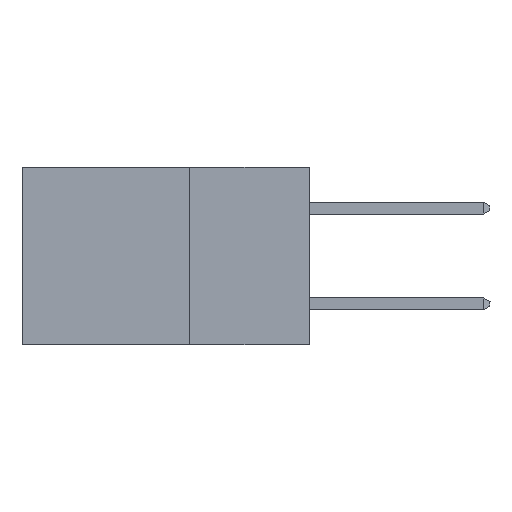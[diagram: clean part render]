
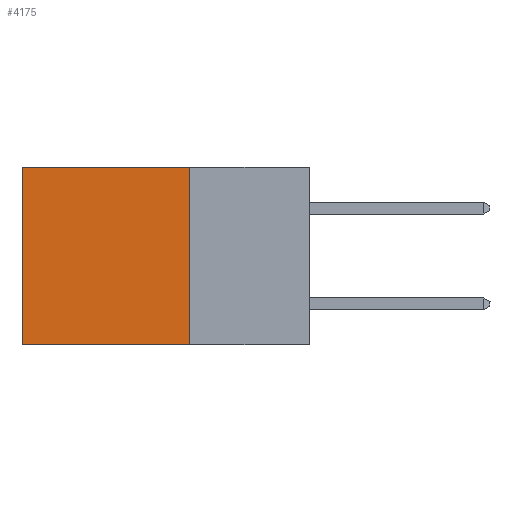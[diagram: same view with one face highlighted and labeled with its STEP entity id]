
A CAD part, left-side view. The second image highlights one B-rep face of the part: STEP entity #4175.
In plain terms, the highlighted planar face has unit normal (-1, 0, 0).
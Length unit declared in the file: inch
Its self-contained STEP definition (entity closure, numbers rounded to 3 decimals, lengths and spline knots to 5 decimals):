
#1829 = LINE ( 'NONE', #14982, #41077 ) ;
#2457 = EDGE_CURVE ( 'NONE', #2562, #21007, #1829, .T. ) ;
#2562 = VERTEX_POINT ( 'NONE', #29993 ) ;
#2972 = VERTEX_POINT ( 'NONE', #21558 ) ;
#3708 = DIRECTION ( 'NONE',  ( 0., 0., -1. ) ) ;
#4175 = ADVANCED_FACE ( 'NONE', ( #35116 ), #12859, .F. ) ;
#5613 = VECTOR ( 'NONE', #24738, 39.37008 ) ;
#9322 = EDGE_CURVE ( 'NONE', #2562, #31354, #25242, .T. ) ;
#9738 = DIRECTION ( 'NONE',  ( 1., 0., 0. ) ) ;
#10698 = CARTESIAN_POINT ( 'NONE',  ( 0.2875, 0.25, -0.37 ) ) ;
#11282 = LINE ( 'NONE', #33806, #42014 ) ;
#12859 = PLANE ( 'NONE',  #41239 ) ;
#13167 = LINE ( 'NONE', #10698, #26453 ) ;
#13308 = DIRECTION ( 'NONE',  ( 0., 0., -1. ) ) ;
#13488 = ORIENTED_EDGE ( 'NONE', *, *, #2457, .T. ) ;
#14982 = CARTESIAN_POINT ( 'NONE',  ( 0.2875, 0.25, 0. ) ) ;
#16525 = ORIENTED_EDGE ( 'NONE', *, *, #23490, .F. ) ;
#17623 = EDGE_CURVE ( 'NONE', #21007, #2972, #11282, .T. ) ;
#18152 = ORIENTED_EDGE ( 'NONE', *, *, #9322, .F. ) ;
#18176 = CARTESIAN_POINT ( 'NONE',  ( 0.2875, 0.25, -0.37 ) ) ;
#19420 = CARTESIAN_POINT ( 'NONE',  ( 0.2875, 0.25, 0. ) ) ;
#20491 = ORIENTED_EDGE ( 'NONE', *, *, #17623, .T. ) ;
#21007 = VERTEX_POINT ( 'NONE', #39632 ) ;
#21558 = CARTESIAN_POINT ( 'NONE',  ( 0.2875, 0.6, -0.37 ) ) ;
#23490 = EDGE_CURVE ( 'NONE', #31354, #2972, #13167, .T. ) ;
#24738 = DIRECTION ( 'NONE',  ( 0., 0., -1. ) ) ;
#25242 = LINE ( 'NONE', #42061, #5613 ) ;
#26453 = VECTOR ( 'NONE', #34866, 39.37008 ) ;
#29993 = CARTESIAN_POINT ( 'NONE',  ( 0.2875, 0.25, 0. ) ) ;
#31354 = VERTEX_POINT ( 'NONE', #18176 ) ;
#31563 = DIRECTION ( 'NONE',  ( 0., 1., 0. ) ) ;
#33806 = CARTESIAN_POINT ( 'NONE',  ( 0.2875, 0.6, 0. ) ) ;
#34711 = EDGE_LOOP ( 'NONE', ( #20491, #16525, #18152, #13488 ) ) ;
#34866 = DIRECTION ( 'NONE',  ( 0., 1., 0. ) ) ;
#35116 = FACE_OUTER_BOUND ( 'NONE', #34711, .T. ) ;
#39632 = CARTESIAN_POINT ( 'NONE',  ( 0.2875, 0.6, 0. ) ) ;
#41077 = VECTOR ( 'NONE', #31563, 39.37008 ) ;
#41239 = AXIS2_PLACEMENT_3D ( 'NONE', #19420, #9738, #13308 ) ;
#42014 = VECTOR ( 'NONE', #3708, 39.37008 ) ;
#42061 = CARTESIAN_POINT ( 'NONE',  ( 0.2875, 0.25, 0. ) ) ;
